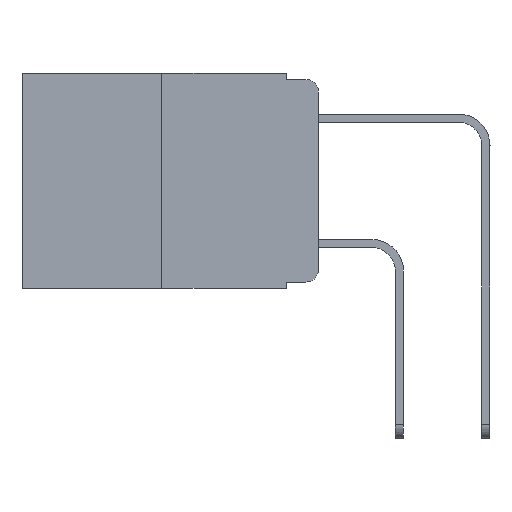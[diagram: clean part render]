
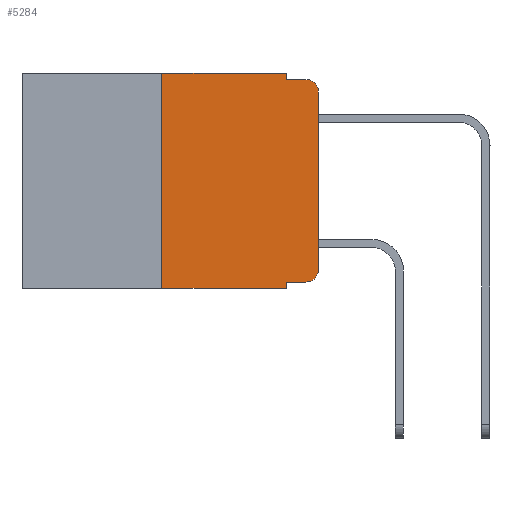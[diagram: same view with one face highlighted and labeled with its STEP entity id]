
A CAD part, left-side view. The second image highlights one B-rep face of the part: STEP entity #5284.
In plain terms, the highlighted planar face has unit normal (-1, 0, 0).
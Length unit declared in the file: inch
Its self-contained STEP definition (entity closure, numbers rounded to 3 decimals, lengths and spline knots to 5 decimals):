
#209 = VECTOR ( 'NONE', #7189, 39.37008 ) ;
#345 = ORIENTED_EDGE ( 'NONE', *, *, #13270, .F. ) ;
#480 = FACE_OUTER_BOUND ( 'NONE', #6962, .T. ) ;
#535 = DIRECTION ( 'NONE',  ( -1., 0., 0. ) ) ;
#802 = LINE ( 'NONE', #11577, #6727 ) ;
#917 = CARTESIAN_POINT ( 'NONE',  ( 0., 0.051, -0.333 ) ) ;
#1409 = VERTEX_POINT ( 'NONE', #15360 ) ;
#1483 = AXIS2_PLACEMENT_3D ( 'NONE', #3126, #535, #11890 ) ;
#1709 = EDGE_CURVE ( 'NONE', #5993, #15498, #6586, .T. ) ;
#1729 = CARTESIAN_POINT ( 'NONE',  ( 0., 0.051, 0. ) ) ;
#1768 = ORIENTED_EDGE ( 'NONE', *, *, #12645, .F. ) ;
#1914 = CARTESIAN_POINT ( 'NONE',  ( 0., 0.051, 0. ) ) ;
#2095 = ORIENTED_EDGE ( 'NONE', *, *, #14083, .T. ) ;
#2226 = DIRECTION ( 'NONE',  ( 1., 0., 0. ) ) ;
#2494 = AXIS2_PLACEMENT_3D ( 'NONE', #9650, #2226, #5863 ) ;
#2498 = ORIENTED_EDGE ( 'NONE', *, *, #10064, .F. ) ;
#2553 = EDGE_CURVE ( 'NONE', #14316, #2565, #5503, .T. ) ;
#2554 = ORIENTED_EDGE ( 'NONE', *, *, #5237, .T. ) ;
#2565 = VERTEX_POINT ( 'NONE', #12170 ) ;
#2768 = EDGE_CURVE ( 'NONE', #9461, #1409, #12712, .T. ) ;
#2857 = CIRCLE ( 'NONE', #4177, 0.02 ) ;
#3126 = CARTESIAN_POINT ( 'NONE',  ( 0., 0.02, -0.03 ) ) ;
#3394 = CARTESIAN_POINT ( 'NONE',  ( 0., 0.473, 0. ) ) ;
#3628 = ORIENTED_EDGE ( 'NONE', *, *, #3948, .T. ) ;
#3948 = EDGE_CURVE ( 'NONE', #15278, #11310, #12488, .T. ) ;
#4011 = CARTESIAN_POINT ( 'NONE',  ( 0., 0.051, -0.01 ) ) ;
#4177 = AXIS2_PLACEMENT_3D ( 'NONE', #7863, #5505, #15393 ) ;
#4925 = VECTOR ( 'NONE', #9573, 39.37008 ) ;
#5185 = VERTEX_POINT ( 'NONE', #14304 ) ;
#5237 = EDGE_CURVE ( 'NONE', #1409, #15278, #2857, .T. ) ;
#5284 = ADVANCED_FACE ( 'NONE', ( #480 ), #7188, .F. ) ;
#5419 = VECTOR ( 'NONE', #12204, 39.37008 ) ;
#5503 = LINE ( 'NONE', #15735, #4925 ) ;
#5505 = DIRECTION ( 'NONE',  ( -1., 0., 0. ) ) ;
#5518 = CARTESIAN_POINT ( 'NONE',  ( 0., 0., -0.313 ) ) ;
#5863 = DIRECTION ( 'NONE',  ( 0., 0., -1. ) ) ;
#5911 = ORIENTED_EDGE ( 'NONE', *, *, #1709, .F. ) ;
#5993 = VERTEX_POINT ( 'NONE', #1729 ) ;
#6397 = ORIENTED_EDGE ( 'NONE', *, *, #2768, .T. ) ;
#6586 = LINE ( 'NONE', #12311, #5419 ) ;
#6727 = VECTOR ( 'NONE', #7785, 39.37008 ) ;
#6945 = LINE ( 'NONE', #15195, #14968 ) ;
#6962 = EDGE_LOOP ( 'NONE', ( #3628, #2095, #345, #5911, #7304, #1768, #11169, #2498, #6397, #2554 ) ) ;
#7188 = PLANE ( 'NONE',  #2494 ) ;
#7189 = DIRECTION ( 'NONE',  ( 0., -1., 0. ) ) ;
#7304 = ORIENTED_EDGE ( 'NONE', *, *, #10780, .F. ) ;
#7785 = DIRECTION ( 'NONE',  ( 0., -1., 0. ) ) ;
#7863 = CARTESIAN_POINT ( 'NONE',  ( 0., 0.02, -0.313 ) ) ;
#8193 = DIRECTION ( 'NONE',  ( 0., 0., 1. ) ) ;
#8266 = CARTESIAN_POINT ( 'NONE',  ( 0., 0., -0.03 ) ) ;
#8321 = VECTOR ( 'NONE', #13154, 39.37008 ) ;
#8349 = CARTESIAN_POINT ( 'NONE',  ( 0., 0.051, -0.333 ) ) ;
#9368 = CARTESIAN_POINT ( 'NONE',  ( 0., 0., 0. ) ) ;
#9461 = VERTEX_POINT ( 'NONE', #8349 ) ;
#9573 = DIRECTION ( 'NONE',  ( 0., -1., 0. ) ) ;
#9614 = CARTESIAN_POINT ( 'NONE',  ( 0., 0.02, -0.01 ) ) ;
#9650 = CARTESIAN_POINT ( 'NONE',  ( 0., 0.473, 0. ) ) ;
#10064 = EDGE_CURVE ( 'NONE', #9461, #2565, #13963, .T. ) ;
#10780 = EDGE_CURVE ( 'NONE', #5185, #5993, #14356, .T. ) ;
#11143 = DIRECTION ( 'NONE',  ( 0., -1., 0. ) ) ;
#11169 = ORIENTED_EDGE ( 'NONE', *, *, #2553, .T. ) ;
#11310 = VERTEX_POINT ( 'NONE', #8266 ) ;
#11567 = CIRCLE ( 'NONE', #1483, 0.02 ) ;
#11577 = CARTESIAN_POINT ( 'NONE',  ( 0., 0.051, -0.01 ) ) ;
#11890 = DIRECTION ( 'NONE',  ( 0., 0., -1. ) ) ;
#12170 = CARTESIAN_POINT ( 'NONE',  ( 0., 0.051, -0.343 ) ) ;
#12204 = DIRECTION ( 'NONE',  ( 0., 0., -1. ) ) ;
#12311 = CARTESIAN_POINT ( 'NONE',  ( 0., 0.051, 0. ) ) ;
#12488 = LINE ( 'NONE', #9368, #15416 ) ;
#12628 = DIRECTION ( 'NONE',  ( 0., 0., 1. ) ) ;
#12645 = EDGE_CURVE ( 'NONE', #14316, #5185, #6945, .T. ) ;
#12712 = LINE ( 'NONE', #917, #13898 ) ;
#13154 = DIRECTION ( 'NONE',  ( 0., 0., -1. ) ) ;
#13270 = EDGE_CURVE ( 'NONE', #15498, #15776, #802, .T. ) ;
#13898 = VECTOR ( 'NONE', #11143, 39.37008 ) ;
#13963 = LINE ( 'NONE', #1914, #8321 ) ;
#14083 = EDGE_CURVE ( 'NONE', #11310, #15776, #11567, .T. ) ;
#14304 = CARTESIAN_POINT ( 'NONE',  ( 0., 0.25, 0. ) ) ;
#14316 = VERTEX_POINT ( 'NONE', #14854 ) ;
#14356 = LINE ( 'NONE', #3394, #209 ) ;
#14854 = CARTESIAN_POINT ( 'NONE',  ( 0., 0.25, -0.343 ) ) ;
#14968 = VECTOR ( 'NONE', #12628, 39.37008 ) ;
#15195 = CARTESIAN_POINT ( 'NONE',  ( 0., 0.25, 0. ) ) ;
#15278 = VERTEX_POINT ( 'NONE', #5518 ) ;
#15360 = CARTESIAN_POINT ( 'NONE',  ( 0., 0.02, -0.333 ) ) ;
#15393 = DIRECTION ( 'NONE',  ( 0., 0., -1. ) ) ;
#15416 = VECTOR ( 'NONE', #8193, 39.37008 ) ;
#15498 = VERTEX_POINT ( 'NONE', #4011 ) ;
#15735 = CARTESIAN_POINT ( 'NONE',  ( 0., 0.473, -0.343 ) ) ;
#15776 = VERTEX_POINT ( 'NONE', #9614 ) ;
